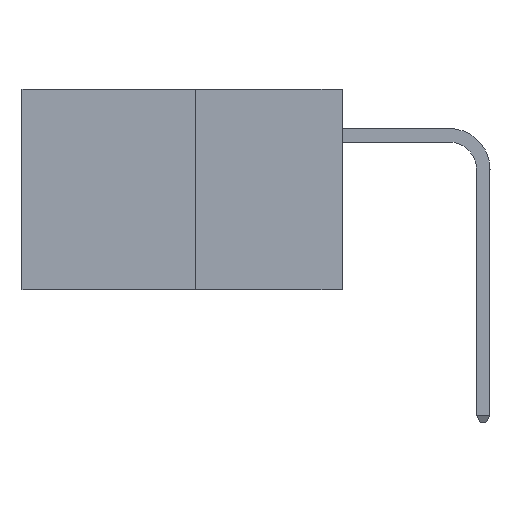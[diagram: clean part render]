
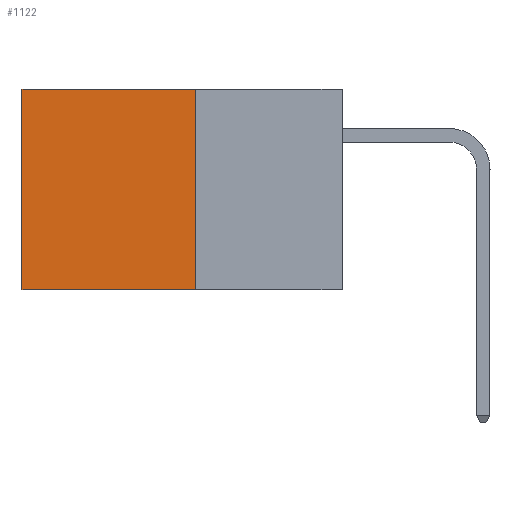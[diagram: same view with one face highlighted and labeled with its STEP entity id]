
A CAD part, left-side view. The second image highlights one B-rep face of the part: STEP entity #1122.
In plain terms, the highlighted planar face has unit normal (-1, 0, 0).
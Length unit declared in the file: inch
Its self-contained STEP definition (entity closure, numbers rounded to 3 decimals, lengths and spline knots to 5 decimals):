
#524 = EDGE_CURVE ( 'NONE', #11925, #6284, #1104, .T. ) ;
#726 = CARTESIAN_POINT ( 'NONE',  ( 0.277, 0.27, 0. ) ) ;
#812 = VECTOR ( 'NONE', #11972, 39.37008 ) ;
#938 = PLANE ( 'NONE',  #12235 ) ;
#1087 = ORIENTED_EDGE ( 'NONE', *, *, #524, .F. ) ;
#1104 = LINE ( 'NONE', #6221, #812 ) ;
#1122 = ADVANCED_FACE ( 'NONE', ( #1397 ), #938, .F. ) ;
#1397 = FACE_OUTER_BOUND ( 'NONE', #11554, .T. ) ;
#1733 = EDGE_CURVE ( 'NONE', #12238, #5741, #10760, .T. ) ;
#2332 = EDGE_CURVE ( 'NONE', #5741, #6284, #11831, .T. ) ;
#2467 = CARTESIAN_POINT ( 'NONE',  ( 0.277, 0.27, -0.37 ) ) ;
#2730 = DIRECTION ( 'NONE',  ( 0., 0., -1. ) ) ;
#3077 = CARTESIAN_POINT ( 'NONE',  ( 0.277, 0.59, -0.37 ) ) ;
#3139 = VECTOR ( 'NONE', #2730, 39.37008 ) ;
#3206 = CARTESIAN_POINT ( 'NONE',  ( 0.277, 0.27, -0.37 ) ) ;
#3270 = VECTOR ( 'NONE', #11238, 39.37008 ) ;
#5098 = EDGE_CURVE ( 'NONE', #12238, #11925, #10379, .T. ) ;
#5239 = CARTESIAN_POINT ( 'NONE',  ( 0.277, 0.27, -0.37 ) ) ;
#5738 = DIRECTION ( 'NONE',  ( 0., 0., -1. ) ) ;
#5741 = VERTEX_POINT ( 'NONE', #6644 ) ;
#6221 = CARTESIAN_POINT ( 'NONE',  ( 0.277, 0.27, -0.37 ) ) ;
#6284 = VERTEX_POINT ( 'NONE', #3077 ) ;
#6373 = ORIENTED_EDGE ( 'NONE', *, *, #5098, .F. ) ;
#6644 = CARTESIAN_POINT ( 'NONE',  ( 0.277, 0.59, 0. ) ) ;
#6757 = VECTOR ( 'NONE', #12093, 39.37008 ) ;
#9149 = CARTESIAN_POINT ( 'NONE',  ( 0.277, 0.27, 0. ) ) ;
#10379 = LINE ( 'NONE', #2467, #3139 ) ;
#10760 = LINE ( 'NONE', #726, #3270 ) ;
#10955 = ORIENTED_EDGE ( 'NONE', *, *, #2332, .T. ) ;
#11238 = DIRECTION ( 'NONE',  ( 0., 1., 0. ) ) ;
#11242 = ORIENTED_EDGE ( 'NONE', *, *, #1733, .T. ) ;
#11269 = DIRECTION ( 'NONE',  ( 1., 0., 0. ) ) ;
#11554 = EDGE_LOOP ( 'NONE', ( #10955, #1087, #6373, #11242 ) ) ;
#11579 = CARTESIAN_POINT ( 'NONE',  ( 0.277, 0.59, -0.37 ) ) ;
#11831 = LINE ( 'NONE', #11579, #6757 ) ;
#11925 = VERTEX_POINT ( 'NONE', #3206 ) ;
#11972 = DIRECTION ( 'NONE',  ( 0., 1., 0. ) ) ;
#12093 = DIRECTION ( 'NONE',  ( 0., 0., -1. ) ) ;
#12235 = AXIS2_PLACEMENT_3D ( 'NONE', #5239, #11269, #5738 ) ;
#12238 = VERTEX_POINT ( 'NONE', #9149 ) ;
